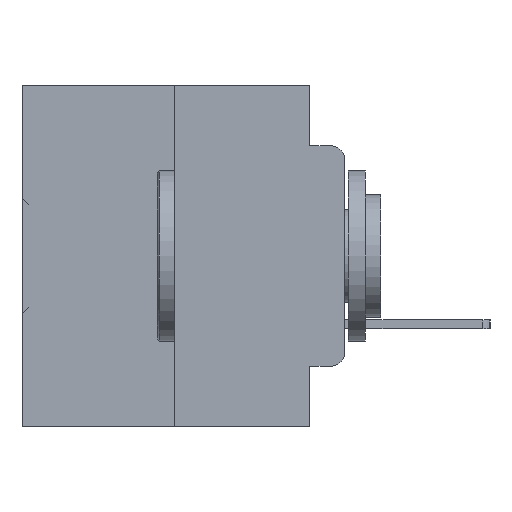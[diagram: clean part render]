
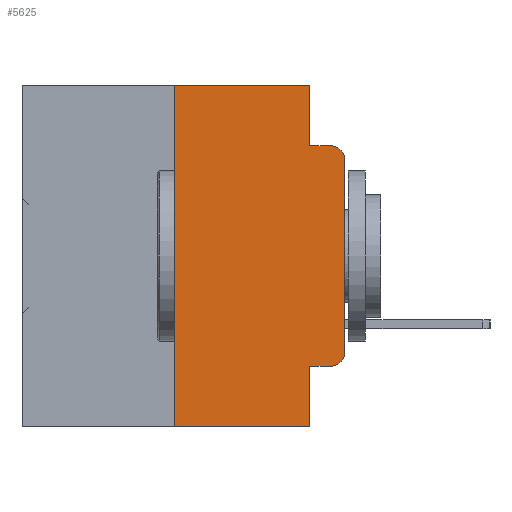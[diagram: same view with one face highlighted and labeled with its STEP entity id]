
A CAD part, left-side view. The second image highlights one B-rep face of the part: STEP entity #5625.
In plain terms, the highlighted planar face has unit normal (-1, 0, 0).
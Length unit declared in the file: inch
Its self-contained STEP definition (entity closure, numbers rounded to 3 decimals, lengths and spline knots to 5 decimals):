
#167 = CARTESIAN_POINT ( 'NONE',  ( 0., 0.051, -0.5 ) ) ;
#273 = CARTESIAN_POINT ( 'NONE',  ( 0., 0.25, 0. ) ) ;
#388 = CARTESIAN_POINT ( 'NONE',  ( 0., 0.051, 0. ) ) ;
#455 = DIRECTION ( 'NONE',  ( -1., 0., 0. ) ) ;
#889 = DIRECTION ( 'NONE',  ( -1., 0., 0. ) ) ;
#1325 = CARTESIAN_POINT ( 'NONE',  ( 0., 0.473, -0.5 ) ) ;
#2853 = DIRECTION ( 'NONE',  ( 0., 0., 1. ) ) ;
#3171 = DIRECTION ( 'NONE',  ( 0., 0., -1. ) ) ;
#3976 = DIRECTION ( 'NONE',  ( 1., 0., 0. ) ) ;
#4103 = LINE ( 'NONE', #8403, #25651 ) ;
#5371 = VECTOR ( 'NONE', #20992, 39.37008 ) ;
#5625 = ADVANCED_FACE ( 'NONE', ( #24787 ), #34555, .F. ) ;
#6663 = VECTOR ( 'NONE', #8080, 39.37008 ) ;
#6786 = VERTEX_POINT ( 'NONE', #10068 ) ;
#7020 = VECTOR ( 'NONE', #17149, 39.37008 ) ;
#7254 = LINE ( 'NONE', #29648, #8152 ) ;
#7784 = CARTESIAN_POINT ( 'NONE',  ( 0., 0.051, -0.0885 ) ) ;
#8080 = DIRECTION ( 'NONE',  ( 0., -1., 0. ) ) ;
#8152 = VECTOR ( 'NONE', #10144, 39.37008 ) ;
#8397 = EDGE_CURVE ( 'NONE', #32551, #34556, #23322, .T. ) ;
#8403 = CARTESIAN_POINT ( 'NONE',  ( 0., 0.473, 0. ) ) ;
#10019 = VECTOR ( 'NONE', #3171, 39.37008 ) ;
#10068 = CARTESIAN_POINT ( 'NONE',  ( 0., 0.051, -0.4115 ) ) ;
#10144 = DIRECTION ( 'NONE',  ( 0., 0., -1. ) ) ;
#11371 = CARTESIAN_POINT ( 'NONE',  ( 0., 0.25, 0. ) ) ;
#11600 = EDGE_LOOP ( 'NONE', ( #25667, #15211, #35074, #32103, #20013, #16113, #30821, #17875, #28758, #29604 ) ) ;
#12145 = EDGE_CURVE ( 'NONE', #6786, #32551, #14145, .T. ) ;
#13814 = LINE ( 'NONE', #7784, #35872 ) ;
#14145 = LINE ( 'NONE', #24878, #6663 ) ;
#14501 = LINE ( 'NONE', #273, #7020 ) ;
#15156 = VERTEX_POINT ( 'NONE', #11371 ) ;
#15211 = ORIENTED_EDGE ( 'NONE', *, *, #27150, .T. ) ;
#15620 = VERTEX_POINT ( 'NONE', #167 ) ;
#15939 = EDGE_CURVE ( 'NONE', #6786, #15620, #7254, .T. ) ;
#16113 = ORIENTED_EDGE ( 'NONE', *, *, #19660, .F. ) ;
#16209 = EDGE_CURVE ( 'NONE', #15156, #16430, #4103, .T. ) ;
#16430 = VERTEX_POINT ( 'NONE', #23462 ) ;
#17149 = DIRECTION ( 'NONE',  ( 0., 0., 1. ) ) ;
#17325 = CARTESIAN_POINT ( 'NONE',  ( 0., 0.02, -0.3915 ) ) ;
#17493 = LINE ( 'NONE', #388, #10019 ) ;
#17764 = CARTESIAN_POINT ( 'NONE',  ( 0., 0.02, -0.1085 ) ) ;
#17875 = ORIENTED_EDGE ( 'NONE', *, *, #15939, .F. ) ;
#18056 = CARTESIAN_POINT ( 'NONE',  ( 0., 0.473, 0. ) ) ;
#18737 = LINE ( 'NONE', #19724, #35110 ) ;
#19660 = EDGE_CURVE ( 'NONE', #29562, #15156, #14501, .T. ) ;
#19724 = CARTESIAN_POINT ( 'NONE',  ( 0., 0., 0. ) ) ;
#20013 = ORIENTED_EDGE ( 'NONE', *, *, #16209, .F. ) ;
#20119 = DIRECTION ( 'NONE',  ( 0., 0., -1. ) ) ;
#20555 = DIRECTION ( 'NONE',  ( 0., 0., -1. ) ) ;
#20992 = DIRECTION ( 'NONE',  ( 0., -1., 0. ) ) ;
#21247 = LINE ( 'NONE', #1325, #5371 ) ;
#21299 = AXIS2_PLACEMENT_3D ( 'NONE', #18056, #3976, #23662 ) ;
#21776 = CARTESIAN_POINT ( 'NONE',  ( 0., 0.02, -0.4115 ) ) ;
#22179 = VERTEX_POINT ( 'NONE', #22843 ) ;
#22843 = CARTESIAN_POINT ( 'NONE',  ( 0., 0.051, -0.0885 ) ) ;
#22932 = VERTEX_POINT ( 'NONE', #28982 ) ;
#23322 = CIRCLE ( 'NONE', #34049, 0.02 ) ;
#23430 = EDGE_CURVE ( 'NONE', #16430, #22179, #17493, .T. ) ;
#23462 = CARTESIAN_POINT ( 'NONE',  ( 0., 0.051, 0. ) ) ;
#23662 = DIRECTION ( 'NONE',  ( 0., 0., -1. ) ) ;
#24201 = CIRCLE ( 'NONE', #24643, 0.02 ) ;
#24643 = AXIS2_PLACEMENT_3D ( 'NONE', #17764, #889, #20555 ) ;
#24787 = FACE_OUTER_BOUND ( 'NONE', #11600, .T. ) ;
#24878 = CARTESIAN_POINT ( 'NONE',  ( 0., 0.051, -0.4115 ) ) ;
#25308 = EDGE_CURVE ( 'NONE', #22179, #31626, #13814, .T. ) ;
#25317 = DIRECTION ( 'NONE',  ( 0., -1., 0. ) ) ;
#25651 = VECTOR ( 'NONE', #25317, 39.37008 ) ;
#25667 = ORIENTED_EDGE ( 'NONE', *, *, #29009, .T. ) ;
#25767 = EDGE_CURVE ( 'NONE', #29562, #15620, #21247, .T. ) ;
#26851 = CARTESIAN_POINT ( 'NONE',  ( 0., 0.02, -0.0885 ) ) ;
#27150 = EDGE_CURVE ( 'NONE', #22932, #31626, #24201, .T. ) ;
#27339 = DIRECTION ( 'NONE',  ( 0., -1., 0. ) ) ;
#28758 = ORIENTED_EDGE ( 'NONE', *, *, #12145, .T. ) ;
#28982 = CARTESIAN_POINT ( 'NONE',  ( 0., 0., -0.1085 ) ) ;
#29009 = EDGE_CURVE ( 'NONE', #34556, #22932, #18737, .T. ) ;
#29562 = VERTEX_POINT ( 'NONE', #34958 ) ;
#29604 = ORIENTED_EDGE ( 'NONE', *, *, #8397, .T. ) ;
#29648 = CARTESIAN_POINT ( 'NONE',  ( 0., 0.051, 0. ) ) ;
#30821 = ORIENTED_EDGE ( 'NONE', *, *, #25767, .T. ) ;
#31626 = VERTEX_POINT ( 'NONE', #26851 ) ;
#32103 = ORIENTED_EDGE ( 'NONE', *, *, #23430, .F. ) ;
#32551 = VERTEX_POINT ( 'NONE', #21776 ) ;
#33904 = CARTESIAN_POINT ( 'NONE',  ( 0., 0., -0.3915 ) ) ;
#34049 = AXIS2_PLACEMENT_3D ( 'NONE', #17325, #455, #20119 ) ;
#34555 = PLANE ( 'NONE',  #21299 ) ;
#34556 = VERTEX_POINT ( 'NONE', #33904 ) ;
#34958 = CARTESIAN_POINT ( 'NONE',  ( 0., 0.25, -0.5 ) ) ;
#35074 = ORIENTED_EDGE ( 'NONE', *, *, #25308, .F. ) ;
#35110 = VECTOR ( 'NONE', #2853, 39.37008 ) ;
#35872 = VECTOR ( 'NONE', #27339, 39.37008 ) ;
